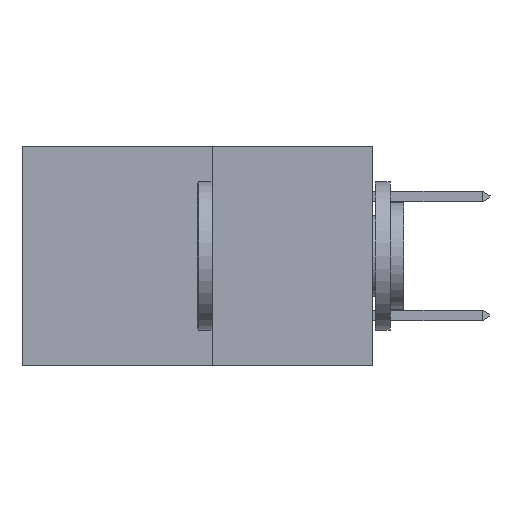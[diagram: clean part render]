
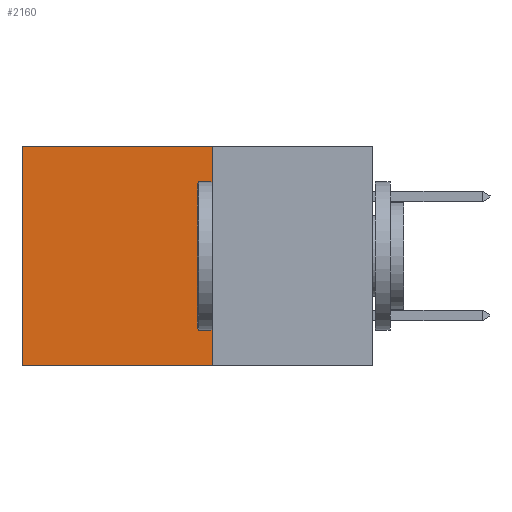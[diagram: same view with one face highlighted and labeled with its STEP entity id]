
A CAD part, left-side view. The second image highlights one B-rep face of the part: STEP entity #2160.
In plain terms, the highlighted planar face has unit normal (-1, 0, 0).
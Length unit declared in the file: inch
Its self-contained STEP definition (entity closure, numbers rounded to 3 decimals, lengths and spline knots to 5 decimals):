
#80 = DIRECTION ( 'NONE',  ( 1., 0., 0. ) ) ;
#153 = AXIS2_PLACEMENT_3D ( 'NONE', #8438, #80, #7455 ) ;
#200 = PLANE ( 'NONE',  #153 ) ;
#205 = VERTEX_POINT ( 'NONE', #4721 ) ;
#454 = VERTEX_POINT ( 'NONE', #5293 ) ;
#616 = DIRECTION ( 'NONE',  ( 0., 0., -1. ) ) ;
#1316 = DIRECTION ( 'NONE',  ( 0., 1., 0. ) ) ;
#1363 = VERTEX_POINT ( 'NONE', #6984 ) ;
#2160 = ADVANCED_FACE ( 'NONE', ( #2218 ), #200, .F. ) ;
#2218 = FACE_OUTER_BOUND ( 'NONE', #6925, .T. ) ;
#3181 = LINE ( 'NONE', #5288, #8757 ) ;
#3573 = CARTESIAN_POINT ( 'NONE',  ( 0.277, 0.27, 0. ) ) ;
#4338 = CARTESIAN_POINT ( 'NONE',  ( 0.277, 0.27, 0. ) ) ;
#4721 = CARTESIAN_POINT ( 'NONE',  ( 0.277, 0.59, 0. ) ) ;
#4919 = ORIENTED_EDGE ( 'NONE', *, *, #6417, .T. ) ;
#5221 = ORIENTED_EDGE ( 'NONE', *, *, #6327, .F. ) ;
#5288 = CARTESIAN_POINT ( 'NONE',  ( 0.277, 0.59, -0.37 ) ) ;
#5293 = CARTESIAN_POINT ( 'NONE',  ( 0.277, 0.27, -0.37 ) ) ;
#5306 = LINE ( 'NONE', #4338, #6986 ) ;
#5341 = ORIENTED_EDGE ( 'NONE', *, *, #7236, .F. ) ;
#5387 = VERTEX_POINT ( 'NONE', #3573 ) ;
#5422 = VECTOR ( 'NONE', #616, 39.37008 ) ;
#5992 = DIRECTION ( 'NONE',  ( 0., 0., -1. ) ) ;
#6119 = EDGE_CURVE ( 'NONE', #5387, #205, #5306, .T. ) ;
#6327 = EDGE_CURVE ( 'NONE', #5387, #454, #7774, .T. ) ;
#6417 = EDGE_CURVE ( 'NONE', #205, #1363, #3181, .T. ) ;
#6925 = EDGE_LOOP ( 'NONE', ( #4919, #5341, #5221, #8025 ) ) ;
#6964 = LINE ( 'NONE', #9430, #8862 ) ;
#6984 = CARTESIAN_POINT ( 'NONE',  ( 0.277, 0.59, -0.37 ) ) ;
#6986 = VECTOR ( 'NONE', #8620, 39.37008 ) ;
#7236 = EDGE_CURVE ( 'NONE', #454, #1363, #6964, .T. ) ;
#7455 = DIRECTION ( 'NONE',  ( 0., 0., -1. ) ) ;
#7774 = LINE ( 'NONE', #9466, #5422 ) ;
#8025 = ORIENTED_EDGE ( 'NONE', *, *, #6119, .T. ) ;
#8438 = CARTESIAN_POINT ( 'NONE',  ( 0.277, 0.27, -0.37 ) ) ;
#8620 = DIRECTION ( 'NONE',  ( 0., 1., 0. ) ) ;
#8757 = VECTOR ( 'NONE', #5992, 39.37008 ) ;
#8862 = VECTOR ( 'NONE', #1316, 39.37008 ) ;
#9430 = CARTESIAN_POINT ( 'NONE',  ( 0.277, 0.27, -0.37 ) ) ;
#9466 = CARTESIAN_POINT ( 'NONE',  ( 0.277, 0.27, -0.37 ) ) ;
